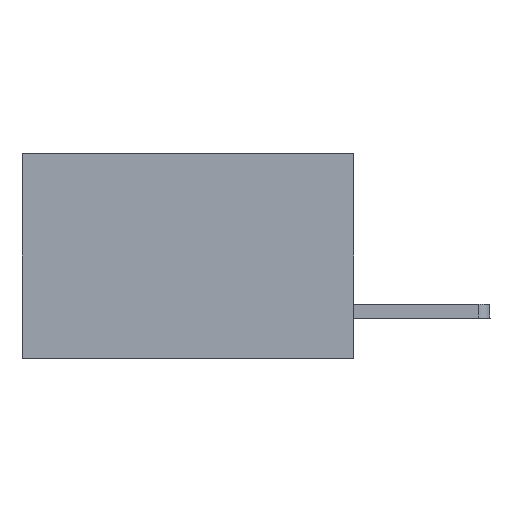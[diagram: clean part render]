
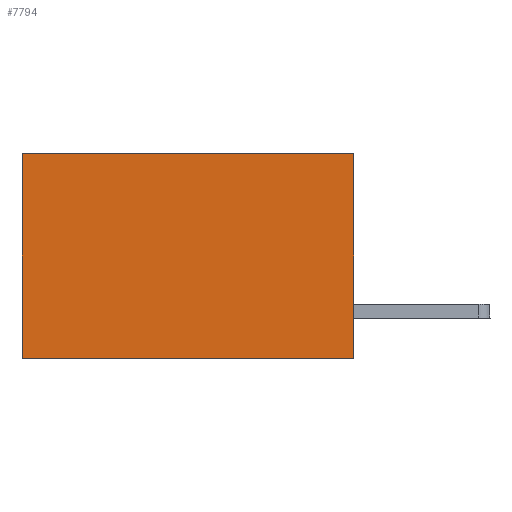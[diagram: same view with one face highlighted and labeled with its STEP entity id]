
A CAD part, left-side view. The second image highlights one B-rep face of the part: STEP entity #7794.
In plain terms, the highlighted planar face has unit normal (-1, 0, 0).
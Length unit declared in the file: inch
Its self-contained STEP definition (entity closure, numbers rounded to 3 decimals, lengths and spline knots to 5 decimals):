
#40 = DIRECTION ( 'NONE',  ( 0., 0., -1. ) ) ;
#587 = CARTESIAN_POINT ( 'NONE',  ( 0.2875, 0., 0. ) ) ;
#1373 = CARTESIAN_POINT ( 'NONE',  ( 0.2875, 0., 0. ) ) ;
#1472 = VERTEX_POINT ( 'NONE', #5334 ) ;
#1588 = VECTOR ( 'NONE', #6612, 39.37008 ) ;
#2592 = LINE ( 'NONE', #6634, #14675 ) ;
#2624 = VERTEX_POINT ( 'NONE', #1373 ) ;
#3306 = VERTEX_POINT ( 'NONE', #3517 ) ;
#3517 = CARTESIAN_POINT ( 'NONE',  ( 0.2875, 0.6, 0. ) ) ;
#3697 = ORIENTED_EDGE ( 'NONE', *, *, #3900, .F. ) ;
#3871 = LINE ( 'NONE', #10395, #15705 ) ;
#3900 = EDGE_CURVE ( 'NONE', #8132, #1472, #12771, .T. ) ;
#5334 = CARTESIAN_POINT ( 'NONE',  ( 0.2875, 0.6, -0.37 ) ) ;
#6127 = DIRECTION ( 'NONE',  ( 0., 1., 0. ) ) ;
#6612 = DIRECTION ( 'NONE',  ( 0., 1., 0. ) ) ;
#6634 = CARTESIAN_POINT ( 'NONE',  ( 0.2875, 0.6, 0. ) ) ;
#6907 = EDGE_CURVE ( 'NONE', #2624, #3306, #8759, .T. ) ;
#6912 = CARTESIAN_POINT ( 'NONE',  ( 0.2875, 0., 0. ) ) ;
#7142 = ORIENTED_EDGE ( 'NONE', *, *, #6907, .T. ) ;
#7620 = EDGE_LOOP ( 'NONE', ( #15480, #3697, #9749, #7142 ) ) ;
#7794 = ADVANCED_FACE ( 'NONE', ( #10372 ), #13930, .F. ) ;
#7871 = CARTESIAN_POINT ( 'NONE',  ( 0.2875, 0., -0.37 ) ) ;
#8108 = DIRECTION ( 'NONE',  ( 0., 0., -1. ) ) ;
#8132 = VERTEX_POINT ( 'NONE', #12191 ) ;
#8318 = EDGE_CURVE ( 'NONE', #3306, #1472, #2592, .T. ) ;
#8759 = LINE ( 'NONE', #587, #1588 ) ;
#8863 = EDGE_CURVE ( 'NONE', #2624, #8132, #3871, .T. ) ;
#9749 = ORIENTED_EDGE ( 'NONE', *, *, #8863, .F. ) ;
#10372 = FACE_OUTER_BOUND ( 'NONE', #7620, .T. ) ;
#10395 = CARTESIAN_POINT ( 'NONE',  ( 0.2875, 0., 0. ) ) ;
#10481 = AXIS2_PLACEMENT_3D ( 'NONE', #6912, #15033, #8108 ) ;
#12191 = CARTESIAN_POINT ( 'NONE',  ( 0.2875, 0., -0.37 ) ) ;
#12715 = DIRECTION ( 'NONE',  ( 0., 0., -1. ) ) ;
#12771 = LINE ( 'NONE', #7871, #15769 ) ;
#13930 = PLANE ( 'NONE',  #10481 ) ;
#14675 = VECTOR ( 'NONE', #40, 39.37008 ) ;
#15033 = DIRECTION ( 'NONE',  ( 1., 0., 0. ) ) ;
#15480 = ORIENTED_EDGE ( 'NONE', *, *, #8318, .T. ) ;
#15705 = VECTOR ( 'NONE', #12715, 39.37008 ) ;
#15769 = VECTOR ( 'NONE', #6127, 39.37008 ) ;
